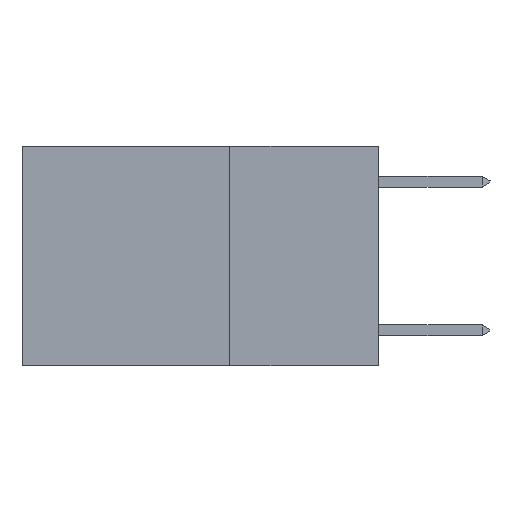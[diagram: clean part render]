
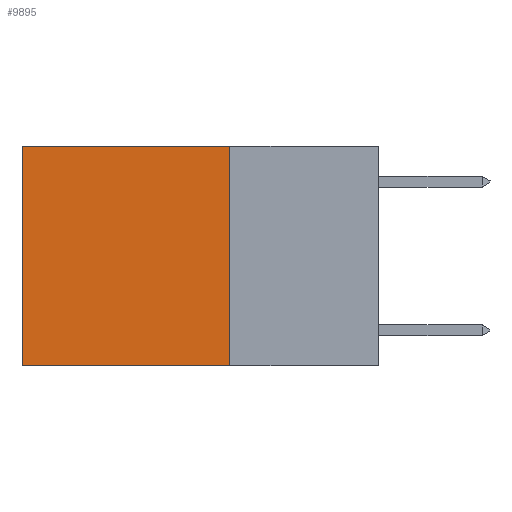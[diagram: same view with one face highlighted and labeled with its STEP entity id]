
A CAD part, left-side view. The second image highlights one B-rep face of the part: STEP entity #9895.
In plain terms, the highlighted planar face has unit normal (-1, 0, 0).
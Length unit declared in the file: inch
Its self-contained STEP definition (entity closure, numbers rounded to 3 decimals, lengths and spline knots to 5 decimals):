
#321 = CARTESIAN_POINT ( 'NONE',  ( 0.2625, 0.6, 0. ) ) ;
#854 = VECTOR ( 'NONE', #2809, 39.37008 ) ;
#1150 = EDGE_CURVE ( 'NONE', #1558, #9439, #9690, .T. ) ;
#1360 = ORIENTED_EDGE ( 'NONE', *, *, #3179, .T. ) ;
#1459 = EDGE_CURVE ( 'NONE', #6028, #1558, #8822, .T. ) ;
#1558 = VERTEX_POINT ( 'NONE', #9649 ) ;
#1709 = VECTOR ( 'NONE', #8373, 39.37008 ) ;
#2091 = FACE_OUTER_BOUND ( 'NONE', #6741, .T. ) ;
#2291 = CARTESIAN_POINT ( 'NONE',  ( 0.2625, 0.25, 0. ) ) ;
#2809 = DIRECTION ( 'NONE',  ( 0., 1., 0. ) ) ;
#2882 = CARTESIAN_POINT ( 'NONE',  ( 0.2625, 0.6, -0.37 ) ) ;
#3179 = EDGE_CURVE ( 'NONE', #4590, #9439, #8169, .T. ) ;
#3187 = DIRECTION ( 'NONE',  ( 0., 1., 0. ) ) ;
#3906 = DIRECTION ( 'NONE',  ( 0., 0., -1. ) ) ;
#4313 = PLANE ( 'NONE',  #9085 ) ;
#4590 = VERTEX_POINT ( 'NONE', #321 ) ;
#5121 = DIRECTION ( 'NONE',  ( 0., 0., -1. ) ) ;
#5193 = CARTESIAN_POINT ( 'NONE',  ( 0.2625, 0.25, 0. ) ) ;
#6028 = VERTEX_POINT ( 'NONE', #5193 ) ;
#6688 = VECTOR ( 'NONE', #3906, 39.37008 ) ;
#6741 = EDGE_LOOP ( 'NONE', ( #1360, #9436, #7509, #6894 ) ) ;
#6832 = CARTESIAN_POINT ( 'NONE',  ( 0.2625, 0.25, -0.37 ) ) ;
#6894 = ORIENTED_EDGE ( 'NONE', *, *, #6943, .T. ) ;
#6943 = EDGE_CURVE ( 'NONE', #6028, #4590, #10432, .T. ) ;
#7509 = ORIENTED_EDGE ( 'NONE', *, *, #1459, .F. ) ;
#7566 = CARTESIAN_POINT ( 'NONE',  ( 0.2625, 0.6, 0. ) ) ;
#8024 = CARTESIAN_POINT ( 'NONE',  ( 0.2625, 0.25, 0. ) ) ;
#8114 = VECTOR ( 'NONE', #3187, 39.37008 ) ;
#8169 = LINE ( 'NONE', #7566, #1709 ) ;
#8306 = CARTESIAN_POINT ( 'NONE',  ( 0.2625, 0.25, 0. ) ) ;
#8373 = DIRECTION ( 'NONE',  ( 0., 0., -1. ) ) ;
#8822 = LINE ( 'NONE', #2291, #6688 ) ;
#9085 = AXIS2_PLACEMENT_3D ( 'NONE', #8306, #9896, #5121 ) ;
#9436 = ORIENTED_EDGE ( 'NONE', *, *, #1150, .F. ) ;
#9439 = VERTEX_POINT ( 'NONE', #2882 ) ;
#9649 = CARTESIAN_POINT ( 'NONE',  ( 0.2625, 0.25, -0.37 ) ) ;
#9690 = LINE ( 'NONE', #6832, #854 ) ;
#9895 = ADVANCED_FACE ( 'NONE', ( #2091 ), #4313, .F. ) ;
#9896 = DIRECTION ( 'NONE',  ( 1., 0., 0. ) ) ;
#10432 = LINE ( 'NONE', #8024, #8114 ) ;
